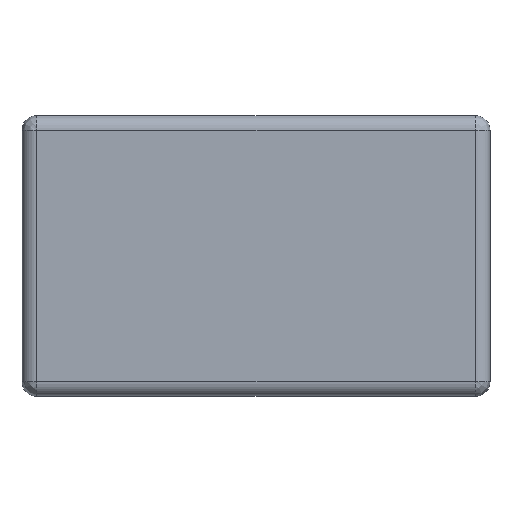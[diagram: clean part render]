
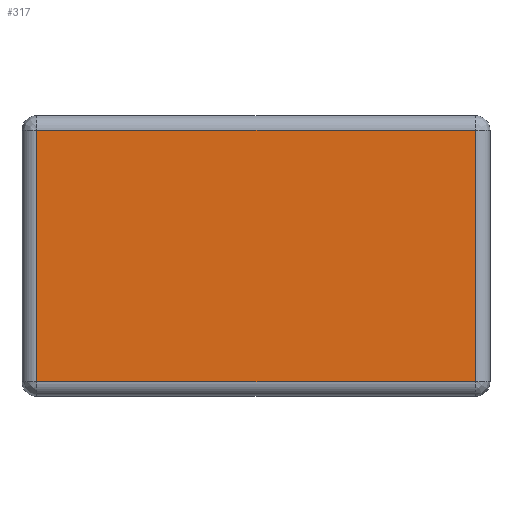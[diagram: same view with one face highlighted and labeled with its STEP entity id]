
A CAD part, top view. The second image highlights one B-rep face of the part: STEP entity #317.
In plain terms, the highlighted planar face has unit normal (0, 0, 1).
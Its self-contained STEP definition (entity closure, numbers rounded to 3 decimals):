
#24 = VERTEX_POINT ( 'NONE', #65 ) ;
#32 = DIRECTION ( 'NONE',  ( 0., -1., 0. ) ) ;
#39 = AXIS2_PLACEMENT_3D ( 'NONE', #115, #343, #81 ) ;
#65 = CARTESIAN_POINT ( 'NONE',  ( 30.75, 1., 3.163 ) ) ;
#75 = DIRECTION ( 'NONE',  ( -1., 0., 0. ) ) ;
#76 = DIRECTION ( 'NONE',  ( 1., 0., 0. ) ) ;
#81 = DIRECTION ( 'NONE',  ( -1., 0., 0. ) ) ;
#115 = CARTESIAN_POINT ( 'NONE',  ( 30.75, 1., 3.163 ) ) ;
#124 = VERTEX_POINT ( 'NONE', #280 ) ;
#133 = ORIENTED_EDGE ( 'NONE', *, *, #179, .F. ) ;
#139 = VERTEX_POINT ( 'NONE', #328 ) ;
#179 = EDGE_CURVE ( 'NONE', #139, #24, #404, .T. ) ;
#222 = EDGE_CURVE ( 'NONE', #392, #139, #347, .T. ) ;
#233 = EDGE_CURVE ( 'NONE', #24, #124, #353, .T. ) ;
#262 = VECTOR ( 'NONE', #466, 1000. ) ;
#272 = FACE_OUTER_BOUND ( 'NONE', #294, .T. ) ;
#280 = CARTESIAN_POINT ( 'NONE',  ( 1., 1., 3.163 ) ) ;
#284 = CARTESIAN_POINT ( 'NONE',  ( 30.75, 9.525, 3.163 ) ) ;
#285 = CARTESIAN_POINT ( 'NONE',  ( 15.875, 1., 3.163 ) ) ;
#291 = PLANE ( 'NONE',  #39 ) ;
#294 = EDGE_LOOP ( 'NONE', ( #446, #501, #524, #133 ) ) ;
#304 = LINE ( 'NONE', #422, #262 ) ;
#311 = EDGE_CURVE ( 'NONE', #392, #124, #304, .T. ) ;
#317 = ADVANCED_FACE ( 'NONE', ( #272 ), #291, .F. ) ;
#328 = CARTESIAN_POINT ( 'NONE',  ( 30.75, 18.05, 3.163 ) ) ;
#332 = VECTOR ( 'NONE', #75, 1000. ) ;
#343 = DIRECTION ( 'NONE',  ( 0., 0., -1. ) ) ;
#347 = LINE ( 'NONE', #505, #364 ) ;
#353 = LINE ( 'NONE', #285, #332 ) ;
#364 = VECTOR ( 'NONE', #76, 1000. ) ;
#386 = VECTOR ( 'NONE', #32, 1000. ) ;
#392 = VERTEX_POINT ( 'NONE', #427 ) ;
#404 = LINE ( 'NONE', #284, #386 ) ;
#422 = CARTESIAN_POINT ( 'NONE',  ( 1., 9.525, 3.162 ) ) ;
#427 = CARTESIAN_POINT ( 'NONE',  ( 1., 18.05, 3.163 ) ) ;
#446 = ORIENTED_EDGE ( 'NONE', *, *, #222, .F. ) ;
#466 = DIRECTION ( 'NONE',  ( 0., -1., 0. ) ) ;
#501 = ORIENTED_EDGE ( 'NONE', *, *, #311, .T. ) ;
#505 = CARTESIAN_POINT ( 'NONE',  ( 15.875, 18.05, 3.163 ) ) ;
#524 = ORIENTED_EDGE ( 'NONE', *, *, #233, .F. ) ;
